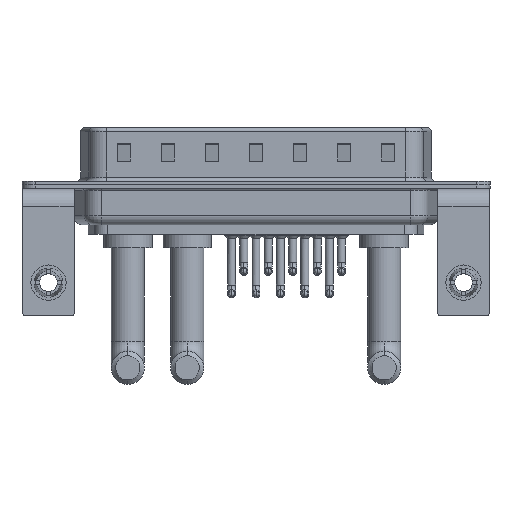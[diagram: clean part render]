
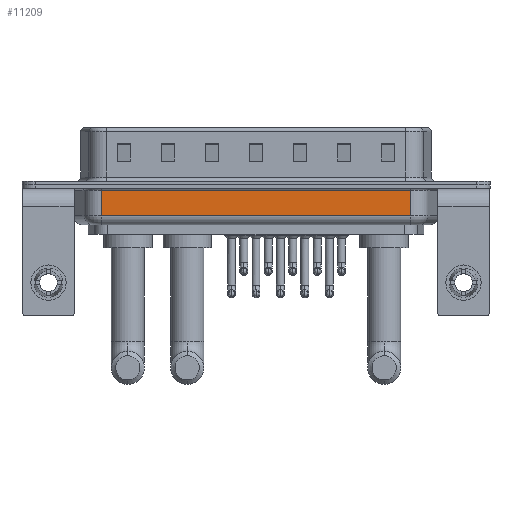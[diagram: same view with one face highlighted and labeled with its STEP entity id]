
A CAD part, front view. The second image highlights one B-rep face of the part: STEP entity #11209.
In plain terms, the highlighted planar face has unit normal (0, -1, 0).
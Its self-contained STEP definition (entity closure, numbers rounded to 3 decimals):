
#8 = VECTOR ( 'NONE', #21554, 1000. ) ;
#1600 = LINE ( 'NONE', #6095, #5387 ) ;
#2456 = DIRECTION ( 'NONE',  ( 0., 0., 1. ) ) ;
#3187 = CARTESIAN_POINT ( 'NONE',  ( 41.044, -5.35, -4.5 ) ) ;
#3947 = VECTOR ( 'NONE', #15329, 1000. ) ;
#4045 = VECTOR ( 'NONE', #16589, 1000. ) ;
#4929 = EDGE_LOOP ( 'NONE', ( #18658, #4983, #21682, #23314 ) ) ;
#4983 = ORIENTED_EDGE ( 'NONE', *, *, #11682, .T. ) ;
#5387 = VECTOR ( 'NONE', #5582, 1000. ) ;
#5582 = DIRECTION ( 'NONE',  ( 1., 0., 0. ) ) ;
#6095 = CARTESIAN_POINT ( 'NONE',  ( 6.006, -5.35, -3.5 ) ) ;
#6695 = CARTESIAN_POINT ( 'NONE',  ( 6.006, -5.35, -4.5 ) ) ;
#8244 = CARTESIAN_POINT ( 'NONE',  ( 41.044, -5.35, -3.5 ) ) ;
#9743 = VERTEX_POINT ( 'NONE', #18307 ) ;
#10259 = FACE_OUTER_BOUND ( 'NONE', #4929, .T. ) ;
#10650 = LINE ( 'NONE', #12756, #4045 ) ;
#11209 = ADVANCED_FACE ( 'NONE', ( #10259 ), #12245, .F. ) ;
#11682 = EDGE_CURVE ( 'NONE', #22989, #25442, #1600, .T. ) ;
#12245 = PLANE ( 'NONE',  #13364 ) ;
#12756 = CARTESIAN_POINT ( 'NONE',  ( 6.006, -5.35, -0.65 ) ) ;
#12764 = DIRECTION ( 'NONE',  ( 0., 1., 0. ) ) ;
#13364 = AXIS2_PLACEMENT_3D ( 'NONE', #6695, #12764, #2456 ) ;
#15207 = LINE ( 'NONE', #25272, #3947 ) ;
#15329 = DIRECTION ( 'NONE',  ( 0., 0., 1. ) ) ;
#16589 = DIRECTION ( 'NONE',  ( -1., 0., 0. ) ) ;
#18307 = CARTESIAN_POINT ( 'NONE',  ( 6.006, -5.35, -0.65 ) ) ;
#18334 = EDGE_CURVE ( 'NONE', #25442, #24577, #25532, .T. ) ;
#18658 = ORIENTED_EDGE ( 'NONE', *, *, #21212, .F. ) ;
#21212 = EDGE_CURVE ( 'NONE', #22989, #9743, #15207, .T. ) ;
#21554 = DIRECTION ( 'NONE',  ( 0., 0., 1. ) ) ;
#21656 = CARTESIAN_POINT ( 'NONE',  ( 6.006, -5.35, -3.5 ) ) ;
#21682 = ORIENTED_EDGE ( 'NONE', *, *, #18334, .T. ) ;
#22421 = EDGE_CURVE ( 'NONE', #24577, #9743, #10650, .T. ) ;
#22989 = VERTEX_POINT ( 'NONE', #21656 ) ;
#23314 = ORIENTED_EDGE ( 'NONE', *, *, #22421, .T. ) ;
#24577 = VERTEX_POINT ( 'NONE', #24601 ) ;
#24601 = CARTESIAN_POINT ( 'NONE',  ( 41.044, -5.35, -0.65 ) ) ;
#25272 = CARTESIAN_POINT ( 'NONE',  ( 6.006, -5.35, -4.5 ) ) ;
#25442 = VERTEX_POINT ( 'NONE', #8244 ) ;
#25532 = LINE ( 'NONE', #3187, #8 ) ;
